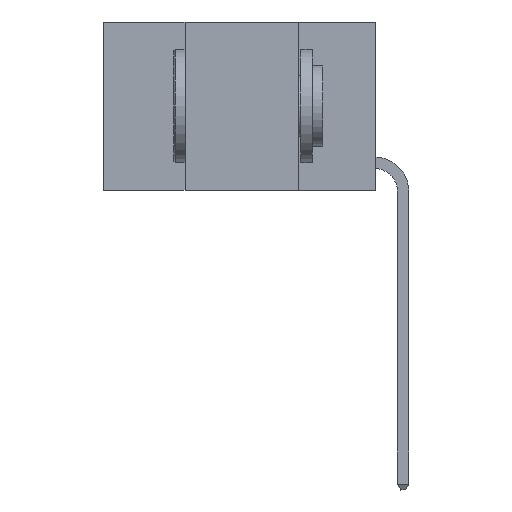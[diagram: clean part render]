
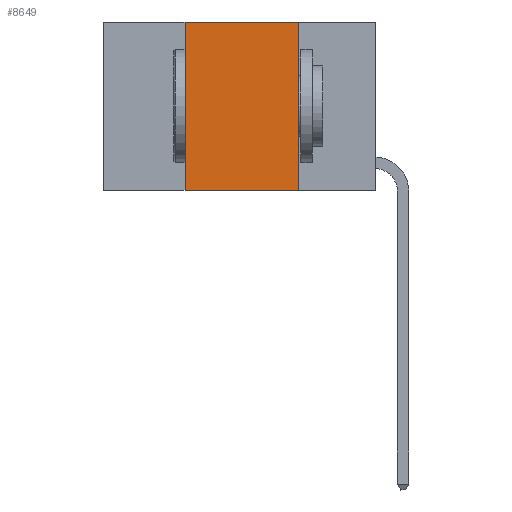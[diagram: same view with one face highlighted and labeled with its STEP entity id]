
A CAD part, left-side view. The second image highlights one B-rep face of the part: STEP entity #8649.
In plain terms, the highlighted planar face has unit normal (-1, 0, 0).
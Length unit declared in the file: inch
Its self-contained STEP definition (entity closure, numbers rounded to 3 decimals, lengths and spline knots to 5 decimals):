
#769 = CARTESIAN_POINT ( 'NONE',  ( 0., 0.17, 0. ) ) ;
#1720 = CARTESIAN_POINT ( 'NONE',  ( 0., 0.6, 0. ) ) ;
#2032 = CARTESIAN_POINT ( 'NONE',  ( 0., 0.6, 0. ) ) ;
#2179 = VECTOR ( 'NONE', #10132, 39.37008 ) ;
#2186 = CARTESIAN_POINT ( 'NONE',  ( 0., 0.42, -0.37 ) ) ;
#2588 = CARTESIAN_POINT ( 'NONE',  ( 0., 0.6, -0.37 ) ) ;
#4291 = AXIS2_PLACEMENT_3D ( 'NONE', #1720, #8054, #18915 ) ;
#4902 = PLANE ( 'NONE',  #4291 ) ;
#5909 = FACE_OUTER_BOUND ( 'NONE', #6517, .T. ) ;
#6107 = VERTEX_POINT ( 'NONE', #14253 ) ;
#6517 = EDGE_LOOP ( 'NONE', ( #15921, #12257, #13578, #14373 ) ) ;
#6698 = DIRECTION ( 'NONE',  ( 0., 0., 1. ) ) ;
#7309 = LINE ( 'NONE', #769, #2179 ) ;
#7463 = LINE ( 'NONE', #14538, #19852 ) ;
#8054 = DIRECTION ( 'NONE',  ( 1., 0., 0. ) ) ;
#8124 = VECTOR ( 'NONE', #18047, 39.37008 ) ;
#8384 = LINE ( 'NONE', #2032, #16200 ) ;
#8649 = ADVANCED_FACE ( 'NONE', ( #5909 ), #4902, .F. ) ;
#10035 = CARTESIAN_POINT ( 'NONE',  ( 0., 0.17, 0. ) ) ;
#10132 = DIRECTION ( 'NONE',  ( 0., 0., -1. ) ) ;
#10652 = VERTEX_POINT ( 'NONE', #2186 ) ;
#10695 = EDGE_CURVE ( 'NONE', #11734, #18143, #7309, .T. ) ;
#11734 = VERTEX_POINT ( 'NONE', #10035 ) ;
#12257 = ORIENTED_EDGE ( 'NONE', *, *, #15786, .F. ) ;
#12310 = LINE ( 'NONE', #2588, #8124 ) ;
#12963 = DIRECTION ( 'NONE',  ( 0., -1., 0. ) ) ;
#13578 = ORIENTED_EDGE ( 'NONE', *, *, #20121, .F. ) ;
#14253 = CARTESIAN_POINT ( 'NONE',  ( 0., 0.42, 0. ) ) ;
#14373 = ORIENTED_EDGE ( 'NONE', *, *, #16024, .T. ) ;
#14538 = CARTESIAN_POINT ( 'NONE',  ( 0., 0.42, 0. ) ) ;
#15615 = CARTESIAN_POINT ( 'NONE',  ( 0., 0.17, -0.37 ) ) ;
#15786 = EDGE_CURVE ( 'NONE', #6107, #11734, #8384, .T. ) ;
#15921 = ORIENTED_EDGE ( 'NONE', *, *, #10695, .F. ) ;
#16024 = EDGE_CURVE ( 'NONE', #10652, #18143, #12310, .T. ) ;
#16200 = VECTOR ( 'NONE', #12963, 39.37008 ) ;
#18047 = DIRECTION ( 'NONE',  ( 0., -1., 0. ) ) ;
#18143 = VERTEX_POINT ( 'NONE', #15615 ) ;
#18915 = DIRECTION ( 'NONE',  ( 0., 0., -1. ) ) ;
#19852 = VECTOR ( 'NONE', #6698, 39.37008 ) ;
#20121 = EDGE_CURVE ( 'NONE', #10652, #6107, #7463, .T. ) ;
